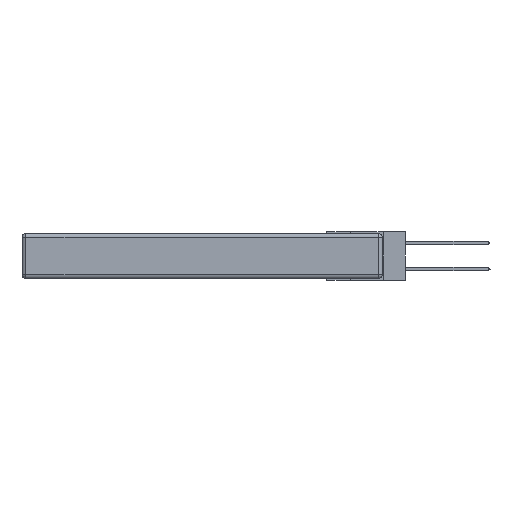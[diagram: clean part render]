
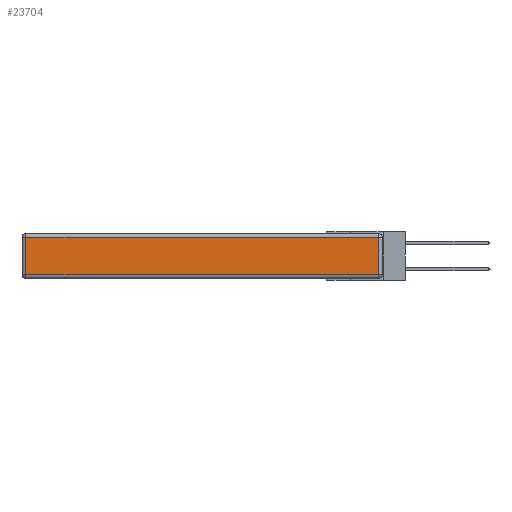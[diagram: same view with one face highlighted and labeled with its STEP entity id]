
A CAD part, left-side view. The second image highlights one B-rep face of the part: STEP entity #23704.
In plain terms, the highlighted planar face has unit normal (-1, 0, 0).
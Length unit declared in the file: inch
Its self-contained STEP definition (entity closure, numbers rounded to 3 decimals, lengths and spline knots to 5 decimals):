
#365 = LINE ( 'NONE', #22816, #19892 ) ;
#741 = CARTESIAN_POINT ( 'NONE',  ( 0., 2.72, -0.03 ) ) ;
#2581 = DIRECTION ( 'NONE',  ( 0., -1., 0. ) ) ;
#3230 = VERTEX_POINT ( 'NONE', #20222 ) ;
#3587 = EDGE_CURVE ( 'NONE', #11637, #3230, #20907, .T. ) ;
#4531 = LINE ( 'NONE', #8460, #23478 ) ;
#4971 = DIRECTION ( 'NONE',  ( 0., 0., 1. ) ) ;
#5165 = ORIENTED_EDGE ( 'NONE', *, *, #5852, .T. ) ;
#5852 = EDGE_CURVE ( 'NONE', #3230, #16494, #4531, .T. ) ;
#6396 = ORIENTED_EDGE ( 'NONE', *, *, #3587, .T. ) ;
#6807 = PLANE ( 'NONE',  #15864 ) ;
#6889 = EDGE_CURVE ( 'NONE', #16494, #18582, #365, .T. ) ;
#8460 = CARTESIAN_POINT ( 'NONE',  ( 0., 0.03, -0.343 ) ) ;
#10442 = DIRECTION ( 'NONE',  ( 0., 0., 1. ) ) ;
#10543 = EDGE_CURVE ( 'NONE', #18582, #11637, #16503, .T. ) ;
#10827 = CARTESIAN_POINT ( 'NONE',  ( 0., 0., -0.343 ) ) ;
#11637 = VERTEX_POINT ( 'NONE', #14076 ) ;
#12756 = EDGE_LOOP ( 'NONE', ( #6396, #5165, #15765, #21489 ) ) ;
#13232 = DIRECTION ( 'NONE',  ( 0., 0., -1. ) ) ;
#13383 = CARTESIAN_POINT ( 'NONE',  ( 0., 2.72, -0.343 ) ) ;
#13949 = CARTESIAN_POINT ( 'NONE',  ( 0., 0., -0.313 ) ) ;
#14076 = CARTESIAN_POINT ( 'NONE',  ( 0., 2.72, -0.313 ) ) ;
#14745 = VECTOR ( 'NONE', #13232, 39.37008 ) ;
#15765 = ORIENTED_EDGE ( 'NONE', *, *, #6889, .T. ) ;
#15864 = AXIS2_PLACEMENT_3D ( 'NONE', #10827, #16320, #4971 ) ;
#16320 = DIRECTION ( 'NONE',  ( -1., 0., 0. ) ) ;
#16494 = VERTEX_POINT ( 'NONE', #18942 ) ;
#16503 = LINE ( 'NONE', #13383, #14745 ) ;
#17273 = DIRECTION ( 'NONE',  ( 0., 1., 0. ) ) ;
#17885 = FACE_OUTER_BOUND ( 'NONE', #12756, .T. ) ;
#18582 = VERTEX_POINT ( 'NONE', #741 ) ;
#18942 = CARTESIAN_POINT ( 'NONE',  ( 0., 0.03, -0.03 ) ) ;
#19892 = VECTOR ( 'NONE', #17273, 39.37008 ) ;
#20222 = CARTESIAN_POINT ( 'NONE',  ( 0., 0.03, -0.313 ) ) ;
#20907 = LINE ( 'NONE', #13949, #22996 ) ;
#21489 = ORIENTED_EDGE ( 'NONE', *, *, #10543, .T. ) ;
#22816 = CARTESIAN_POINT ( 'NONE',  ( 0., 2.75, -0.03 ) ) ;
#22996 = VECTOR ( 'NONE', #2581, 39.37008 ) ;
#23478 = VECTOR ( 'NONE', #10442, 39.37008 ) ;
#23704 = ADVANCED_FACE ( 'NONE', ( #17885 ), #6807, .T. ) ;
